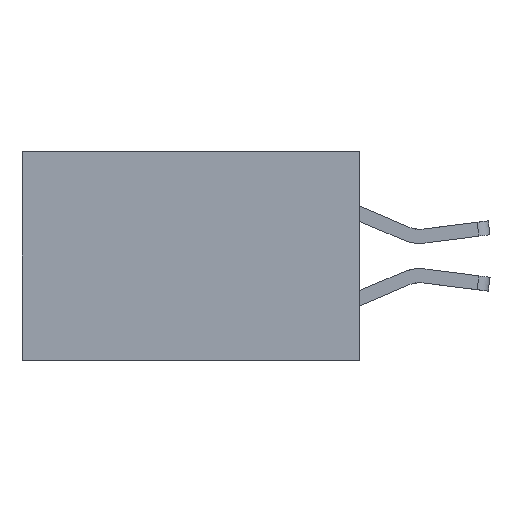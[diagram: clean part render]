
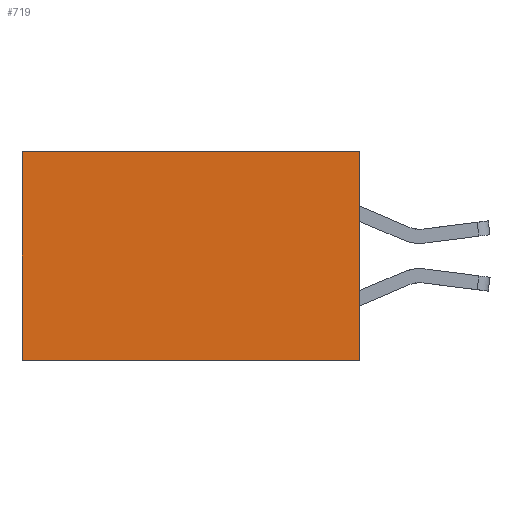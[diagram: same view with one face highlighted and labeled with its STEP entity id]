
A CAD part, left-side view. The second image highlights one B-rep face of the part: STEP entity #719.
In plain terms, the highlighted planar face has unit normal (-1, 0, 0).
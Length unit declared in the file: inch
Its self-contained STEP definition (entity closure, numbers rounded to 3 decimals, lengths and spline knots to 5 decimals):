
#719 = ADVANCED_FACE ( 'NONE', ( #11527 ), #4707, .F. ) ;
#891 = CARTESIAN_POINT ( 'NONE',  ( 0.2875, 0., 0. ) ) ;
#900 = EDGE_CURVE ( 'NONE', #1979, #3923, #4680, .T. ) ;
#931 = ORIENTED_EDGE ( 'NONE', *, *, #900, .T. ) ;
#1287 = ORIENTED_EDGE ( 'NONE', *, *, #11059, .F. ) ;
#1724 = VECTOR ( 'NONE', #11558, 39.37008 ) ;
#1979 = VERTEX_POINT ( 'NONE', #9506 ) ;
#2429 = VECTOR ( 'NONE', #5574, 39.37008 ) ;
#2636 = CARTESIAN_POINT ( 'NONE',  ( 0.2875, 0., -0.37 ) ) ;
#2847 = LINE ( 'NONE', #11908, #4412 ) ;
#3103 = CARTESIAN_POINT ( 'NONE',  ( 0.2875, 0.6, -0.37 ) ) ;
#3413 = CARTESIAN_POINT ( 'NONE',  ( 0.2875, 0., 0. ) ) ;
#3923 = VERTEX_POINT ( 'NONE', #3103 ) ;
#4294 = DIRECTION ( 'NONE',  ( 0., 1., 0. ) ) ;
#4412 = VECTOR ( 'NONE', #4294, 39.37008 ) ;
#4563 = DIRECTION ( 'NONE',  ( 1., 0., 0. ) ) ;
#4589 = ORIENTED_EDGE ( 'NONE', *, *, #11650, .T. ) ;
#4680 = LINE ( 'NONE', #5022, #1724 ) ;
#4707 = PLANE ( 'NONE',  #10032 ) ;
#5022 = CARTESIAN_POINT ( 'NONE',  ( 0.2875, 0.6, 0. ) ) ;
#5544 = VERTEX_POINT ( 'NONE', #2636 ) ;
#5574 = DIRECTION ( 'NONE',  ( 0., 0., -1. ) ) ;
#6633 = VECTOR ( 'NONE', #11846, 39.37008 ) ;
#6634 = ORIENTED_EDGE ( 'NONE', *, *, #11510, .F. ) ;
#9128 = LINE ( 'NONE', #10941, #6633 ) ;
#9220 = EDGE_LOOP ( 'NONE', ( #931, #6634, #1287, #4589 ) ) ;
#9506 = CARTESIAN_POINT ( 'NONE',  ( 0.2875, 0.6, 0. ) ) ;
#9694 = CARTESIAN_POINT ( 'NONE',  ( 0.2875, 0., 0. ) ) ;
#10032 = AXIS2_PLACEMENT_3D ( 'NONE', #9694, #4563, #10401 ) ;
#10267 = VERTEX_POINT ( 'NONE', #891 ) ;
#10378 = LINE ( 'NONE', #3413, #2429 ) ;
#10401 = DIRECTION ( 'NONE',  ( 0., 0., -1. ) ) ;
#10941 = CARTESIAN_POINT ( 'NONE',  ( 0.2875, 0., -0.37 ) ) ;
#11059 = EDGE_CURVE ( 'NONE', #10267, #5544, #10378, .T. ) ;
#11510 = EDGE_CURVE ( 'NONE', #5544, #3923, #9128, .T. ) ;
#11527 = FACE_OUTER_BOUND ( 'NONE', #9220, .T. ) ;
#11558 = DIRECTION ( 'NONE',  ( 0., 0., -1. ) ) ;
#11650 = EDGE_CURVE ( 'NONE', #10267, #1979, #2847, .T. ) ;
#11846 = DIRECTION ( 'NONE',  ( 0., 1., 0. ) ) ;
#11908 = CARTESIAN_POINT ( 'NONE',  ( 0.2875, 0., 0. ) ) ;
